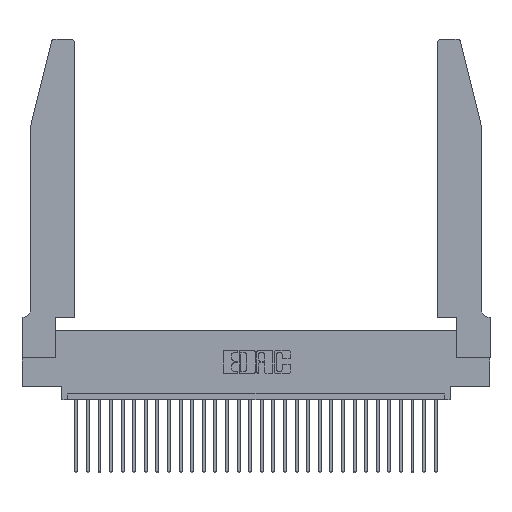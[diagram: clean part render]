
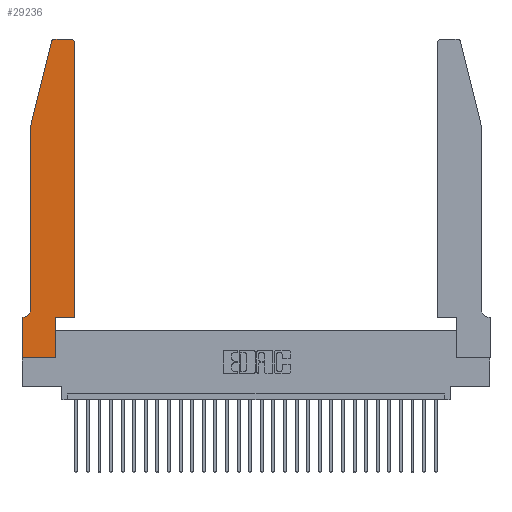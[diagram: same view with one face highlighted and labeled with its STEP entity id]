
A CAD part, top view. The second image highlights one B-rep face of the part: STEP entity #29236.
In plain terms, the highlighted planar face has unit normal (0, 0, 1).
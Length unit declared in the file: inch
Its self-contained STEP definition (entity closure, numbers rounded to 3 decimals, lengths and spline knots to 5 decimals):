
#261 = ORIENTED_EDGE ( 'NONE', *, *, #14808, .T. ) ;
#264 = CARTESIAN_POINT ( 'NONE',  ( 0., 0., 0.37 ) ) ;
#679 = CARTESIAN_POINT ( 'NONE',  ( 0.25487, 2.72718, 0.37 ) ) ;
#697 = EDGE_CURVE ( 'NONE', #19311, #20408, #4402, .T. ) ;
#991 = LINE ( 'NONE', #26334, #19689 ) ;
#1722 = ORIENTED_EDGE ( 'NONE', *, *, #19823, .T. ) ;
#2196 = PLANE ( 'NONE',  #16321 ) ;
#2596 = DIRECTION ( 'NONE',  ( 1., 0., 0. ) ) ;
#3657 = LINE ( 'NONE', #12510, #4409 ) ;
#3759 = ORIENTED_EDGE ( 'NONE', *, *, #697, .T. ) ;
#4217 = DIRECTION ( 'NONE',  ( 0., 1., 0. ) ) ;
#4402 = LINE ( 'NONE', #27123, #13937 ) ;
#4409 = VECTOR ( 'NONE', #5657, 39.37008 ) ;
#4717 = DIRECTION ( 'NONE',  ( -1., 0., 0. ) ) ;
#5337 = EDGE_CURVE ( 'NONE', #29322, #29469, #13769, .T. ) ;
#5568 = DIRECTION ( 'NONE',  ( 0., 0., 1. ) ) ;
#5657 = DIRECTION ( 'NONE',  ( -1., 0., 0. ) ) ;
#6911 = CARTESIAN_POINT ( 'NONE',  ( 0.2865, 0.35, 0.37 ) ) ;
#8718 = EDGE_CURVE ( 'NONE', #18301, #11053, #16154, .T. ) ;
#9295 = CARTESIAN_POINT ( 'NONE',  ( 0.4505, 2.72, 0.37 ) ) ;
#9709 = ORIENTED_EDGE ( 'NONE', *, *, #8718, .T. ) ;
#11053 = VERTEX_POINT ( 'NONE', #22720 ) ;
#11263 = CARTESIAN_POINT ( 'NONE',  ( 0.4505, 0.35, 0.37 ) ) ;
#11396 = CARTESIAN_POINT ( 'NONE',  ( 0.4505, 0.35, 0.37 ) ) ;
#11884 = VERTEX_POINT ( 'NONE', #11263 ) ;
#11901 = DIRECTION ( 'NONE',  ( 0., 0., -1. ) ) ;
#12110 = EDGE_CURVE ( 'NONE', #27243, #24672, #23739, .T. ) ;
#12378 = VECTOR ( 'NONE', #21445, 39.37008 ) ;
#12412 = EDGE_CURVE ( 'NONE', #24672, #18010, #25536, .T. ) ;
#12510 = CARTESIAN_POINT ( 'NONE',  ( 0.2605, 2.75, 0.37 ) ) ;
#12573 = AXIS2_PLACEMENT_3D ( 'NONE', #16144, #20921, #30103 ) ;
#12762 = VERTEX_POINT ( 'NONE', #14651 ) ;
#12806 = CARTESIAN_POINT ( 'NONE',  ( 0.0755, 2., 0.37 ) ) ;
#12901 = DIRECTION ( 'NONE',  ( -0.239, -0.971, 0. ) ) ;
#13165 = EDGE_CURVE ( 'NONE', #20408, #18301, #20828, .T. ) ;
#13329 = CIRCLE ( 'NONE', #15827, 0.07 ) ;
#13769 = CIRCLE ( 'NONE', #12573, 0.03 ) ;
#13793 = DIRECTION ( 'NONE',  ( 0., 0., 1. ) ) ;
#13937 = VECTOR ( 'NONE', #20307, 39.37008 ) ;
#14082 = ORIENTED_EDGE ( 'NONE', *, *, #20131, .T. ) ;
#14285 = CARTESIAN_POINT ( 'NONE',  ( 0., 0., 0.37 ) ) ;
#14479 = CARTESIAN_POINT ( 'NONE',  ( 0.0055, 0.42, 0.37 ) ) ;
#14651 = CARTESIAN_POINT ( 'NONE',  ( 0.284, 2.75, 0.37 ) ) ;
#14808 = EDGE_CURVE ( 'NONE', #12762, #27243, #15977, .T. ) ;
#14959 = VECTOR ( 'NONE', #12901, 39.37008 ) ;
#15025 = CARTESIAN_POINT ( 'NONE',  ( 0.0755, 2., 0.37 ) ) ;
#15468 = CARTESIAN_POINT ( 'NONE',  ( 0.0055, 0.35, 0.37 ) ) ;
#15520 = ORIENTED_EDGE ( 'NONE', *, *, #17196, .T. ) ;
#15694 = CARTESIAN_POINT ( 'NONE',  ( 0.0755, 0.42, 0.37 ) ) ;
#15827 = AXIS2_PLACEMENT_3D ( 'NONE', #14479, #11901, #4717 ) ;
#15977 = CIRCLE ( 'NONE', #16514, 0.03 ) ;
#16144 = CARTESIAN_POINT ( 'NONE',  ( 0.4205, 2.72, 0.37 ) ) ;
#16154 = LINE ( 'NONE', #264, #25611 ) ;
#16321 = AXIS2_PLACEMENT_3D ( 'NONE', #18402, #13793, #30132 ) ;
#16514 = AXIS2_PLACEMENT_3D ( 'NONE', #26609, #5568, #28978 ) ;
#16660 = EDGE_LOOP ( 'NONE', ( #15520, #261, #22215, #24627, #28334, #3759, #23309, #9709, #18576, #14082, #1722, #23014 ) ) ;
#17196 = EDGE_CURVE ( 'NONE', #29469, #12762, #3657, .T. ) ;
#18010 = VERTEX_POINT ( 'NONE', #15694 ) ;
#18301 = VERTEX_POINT ( 'NONE', #30267 ) ;
#18402 = CARTESIAN_POINT ( 'NONE',  ( 0., 0.35, 0.37 ) ) ;
#18576 = ORIENTED_EDGE ( 'NONE', *, *, #22008, .T. ) ;
#18961 = CARTESIAN_POINT ( 'NONE',  ( 0., 0.35, 0.37 ) ) ;
#19311 = VERTEX_POINT ( 'NONE', #15468 ) ;
#19323 = CARTESIAN_POINT ( 'NONE',  ( 0.2865, 0.35, 0.37 ) ) ;
#19332 = VECTOR ( 'NONE', #23727, 39.37008 ) ;
#19535 = VECTOR ( 'NONE', #4217, 39.37008 ) ;
#19689 = VECTOR ( 'NONE', #21785, 39.37008 ) ;
#19823 = EDGE_CURVE ( 'NONE', #11884, #29322, #991, .T. ) ;
#20131 = EDGE_CURVE ( 'NONE', #22756, #11884, #20793, .T. ) ;
#20307 = DIRECTION ( 'NONE',  ( -1., 0., 0. ) ) ;
#20408 = VERTEX_POINT ( 'NONE', #18961 ) ;
#20793 = LINE ( 'NONE', #11396, #30265 ) ;
#20828 = LINE ( 'NONE', #14285, #12378 ) ;
#20921 = DIRECTION ( 'NONE',  ( 0., 0., 1. ) ) ;
#21445 = DIRECTION ( 'NONE',  ( 0., -1., 0. ) ) ;
#21785 = DIRECTION ( 'NONE',  ( 0., 1., 0. ) ) ;
#22008 = EDGE_CURVE ( 'NONE', #11053, #22756, #22850, .T. ) ;
#22215 = ORIENTED_EDGE ( 'NONE', *, *, #12110, .T. ) ;
#22218 = EDGE_CURVE ( 'NONE', #18010, #19311, #13329, .T. ) ;
#22720 = CARTESIAN_POINT ( 'NONE',  ( 0.2865, 0., 0.37 ) ) ;
#22756 = VERTEX_POINT ( 'NONE', #19323 ) ;
#22850 = LINE ( 'NONE', #6911, #19535 ) ;
#23014 = ORIENTED_EDGE ( 'NONE', *, *, #5337, .T. ) ;
#23309 = ORIENTED_EDGE ( 'NONE', *, *, #13165, .T. ) ;
#23727 = DIRECTION ( 'NONE',  ( 0., -1., 0. ) ) ;
#23739 = LINE ( 'NONE', #12806, #14959 ) ;
#23825 = CARTESIAN_POINT ( 'NONE',  ( 0.0755, 2., 0.37 ) ) ;
#24627 = ORIENTED_EDGE ( 'NONE', *, *, #12412, .T. ) ;
#24672 = VERTEX_POINT ( 'NONE', #15025 ) ;
#25536 = LINE ( 'NONE', #23825, #19332 ) ;
#25611 = VECTOR ( 'NONE', #2596, 39.37008 ) ;
#26334 = CARTESIAN_POINT ( 'NONE',  ( 0.4505, 0.35, 0.37 ) ) ;
#26609 = CARTESIAN_POINT ( 'NONE',  ( 0.284, 2.72, 0.37 ) ) ;
#27123 = CARTESIAN_POINT ( 'NONE',  ( 0.0755, 0.35, 0.37 ) ) ;
#27243 = VERTEX_POINT ( 'NONE', #679 ) ;
#27835 = DIRECTION ( 'NONE',  ( 1., 0., 0. ) ) ;
#28334 = ORIENTED_EDGE ( 'NONE', *, *, #22218, .T. ) ;
#28716 = FACE_OUTER_BOUND ( 'NONE', #16660, .T. ) ;
#28881 = CARTESIAN_POINT ( 'NONE',  ( 0.4205, 2.75, 0.37 ) ) ;
#28978 = DIRECTION ( 'NONE',  ( 1., 0., 0. ) ) ;
#29236 = ADVANCED_FACE ( 'NONE', ( #28716 ), #2196, .T. ) ;
#29322 = VERTEX_POINT ( 'NONE', #9295 ) ;
#29469 = VERTEX_POINT ( 'NONE', #28881 ) ;
#30103 = DIRECTION ( 'NONE',  ( 1., 0., 0. ) ) ;
#30132 = DIRECTION ( 'NONE',  ( 1., 0., 0. ) ) ;
#30265 = VECTOR ( 'NONE', #27835, 39.37008 ) ;
#30267 = CARTESIAN_POINT ( 'NONE',  ( 0., 0., 0.37 ) ) ;
